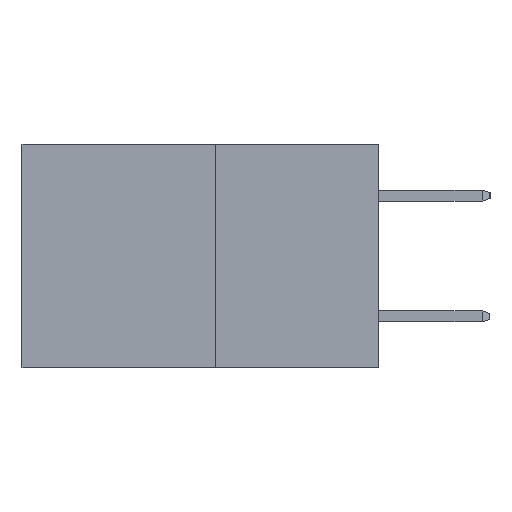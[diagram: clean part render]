
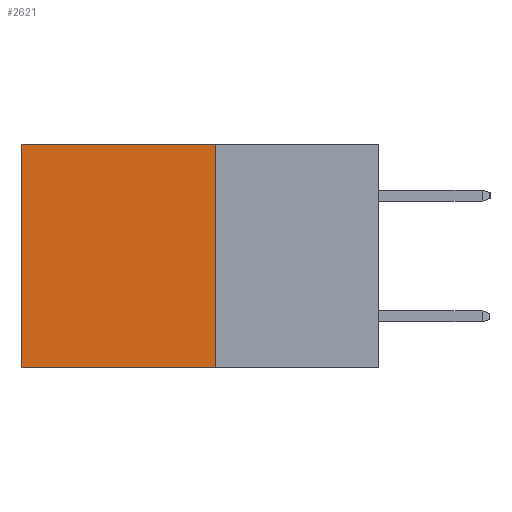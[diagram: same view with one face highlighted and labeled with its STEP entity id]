
A CAD part, left-side view. The second image highlights one B-rep face of the part: STEP entity #2621.
In plain terms, the highlighted planar face has unit normal (-1, 0, 0).
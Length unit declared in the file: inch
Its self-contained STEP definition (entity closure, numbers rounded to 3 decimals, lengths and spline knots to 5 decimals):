
#67 = EDGE_CURVE ( 'NONE', #2740, #9790, #13062, .T. ) ;
#981 = DIRECTION ( 'NONE',  ( 0., 0., -1. ) ) ;
#1136 = ORIENTED_EDGE ( 'NONE', *, *, #2032, .T. ) ;
#1165 = FACE_OUTER_BOUND ( 'NONE', #6837, .T. ) ;
#1261 = VECTOR ( 'NONE', #8929, 39.37008 ) ;
#1896 = LINE ( 'NONE', #5546, #5415 ) ;
#2032 = EDGE_CURVE ( 'NONE', #21973, #10599, #11935, .T. ) ;
#2081 = ORIENTED_EDGE ( 'NONE', *, *, #11443, .T. ) ;
#2621 = ADVANCED_FACE ( 'NONE', ( #1165 ), #12104, .F. ) ;
#2740 = VERTEX_POINT ( 'NONE', #9625 ) ;
#5326 = EDGE_CURVE ( 'NONE', #9790, #10599, #1896, .T. ) ;
#5415 = VECTOR ( 'NONE', #12400, 39.37008 ) ;
#5546 = CARTESIAN_POINT ( 'NONE',  ( 0.277, 0.27, -0.37 ) ) ;
#5587 = AXIS2_PLACEMENT_3D ( 'NONE', #13417, #11985, #11915 ) ;
#6837 = EDGE_LOOP ( 'NONE', ( #1136, #21858, #21413, #2081 ) ) ;
#7228 = CARTESIAN_POINT ( 'NONE',  ( 0.277, 0.27, 0. ) ) ;
#8929 = DIRECTION ( 'NONE',  ( 0., 1., 0. ) ) ;
#9114 = VECTOR ( 'NONE', #981, 39.37008 ) ;
#9625 = CARTESIAN_POINT ( 'NONE',  ( 0.277, 0.27, 0. ) ) ;
#9790 = VERTEX_POINT ( 'NONE', #18795 ) ;
#10361 = DIRECTION ( 'NONE',  ( 0., 0., -1. ) ) ;
#10599 = VERTEX_POINT ( 'NONE', #15131 ) ;
#10844 = CARTESIAN_POINT ( 'NONE',  ( 0.277, 0.59, 0. ) ) ;
#11398 = VECTOR ( 'NONE', #10361, 39.37008 ) ;
#11443 = EDGE_CURVE ( 'NONE', #2740, #21973, #14878, .T. ) ;
#11915 = DIRECTION ( 'NONE',  ( 0., 0., -1. ) ) ;
#11935 = LINE ( 'NONE', #13599, #11398 ) ;
#11985 = DIRECTION ( 'NONE',  ( 1., 0., 0. ) ) ;
#12104 = PLANE ( 'NONE',  #5587 ) ;
#12400 = DIRECTION ( 'NONE',  ( 0., 1., 0. ) ) ;
#13062 = LINE ( 'NONE', #13817, #9114 ) ;
#13417 = CARTESIAN_POINT ( 'NONE',  ( 0.277, 0.27, -0.37 ) ) ;
#13599 = CARTESIAN_POINT ( 'NONE',  ( 0.277, 0.59, -0.37 ) ) ;
#13817 = CARTESIAN_POINT ( 'NONE',  ( 0.277, 0.27, -0.37 ) ) ;
#14878 = LINE ( 'NONE', #7228, #1261 ) ;
#15131 = CARTESIAN_POINT ( 'NONE',  ( 0.277, 0.59, -0.37 ) ) ;
#18795 = CARTESIAN_POINT ( 'NONE',  ( 0.277, 0.27, -0.37 ) ) ;
#21413 = ORIENTED_EDGE ( 'NONE', *, *, #67, .F. ) ;
#21858 = ORIENTED_EDGE ( 'NONE', *, *, #5326, .F. ) ;
#21973 = VERTEX_POINT ( 'NONE', #10844 ) ;
